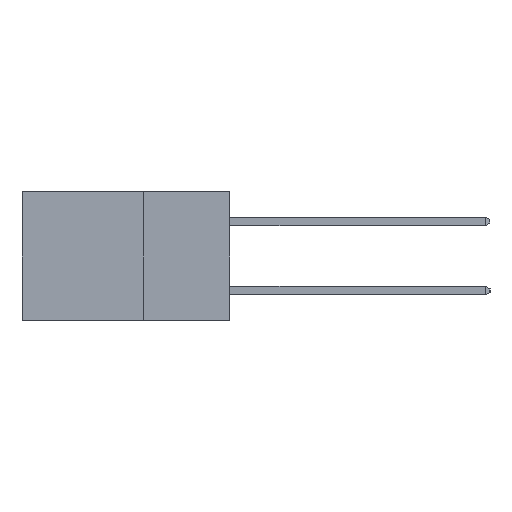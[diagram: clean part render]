
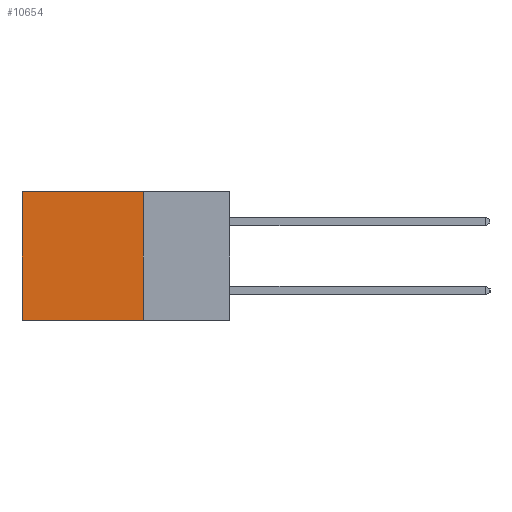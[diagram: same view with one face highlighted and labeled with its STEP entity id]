
A CAD part, left-side view. The second image highlights one B-rep face of the part: STEP entity #10654.
In plain terms, the highlighted planar face has unit normal (-1, 0, 0).
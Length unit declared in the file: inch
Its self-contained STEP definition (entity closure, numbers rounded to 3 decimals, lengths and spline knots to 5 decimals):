
#202 = CARTESIAN_POINT ( 'NONE',  ( 0.2615, 0.25, -0.37 ) ) ;
#442 = DIRECTION ( 'NONE',  ( 0., 0., -1. ) ) ;
#1009 = VERTEX_POINT ( 'NONE', #6782 ) ;
#1456 = DIRECTION ( 'NONE',  ( 1., 0., 0. ) ) ;
#1971 = VECTOR ( 'NONE', #8058, 39.37008 ) ;
#2133 = VERTEX_POINT ( 'NONE', #7729 ) ;
#2610 = CARTESIAN_POINT ( 'NONE',  ( 0.2615, 0.25, -0.37 ) ) ;
#2771 = VECTOR ( 'NONE', #12347, 39.37008 ) ;
#2778 = ORIENTED_EDGE ( 'NONE', *, *, #12112, .F. ) ;
#3104 = VECTOR ( 'NONE', #442, 39.37008 ) ;
#4821 = EDGE_CURVE ( 'NONE', #2133, #5373, #10123, .T. ) ;
#4939 = LINE ( 'NONE', #8272, #1971 ) ;
#5373 = VERTEX_POINT ( 'NONE', #10632 ) ;
#5421 = ORIENTED_EDGE ( 'NONE', *, *, #9676, .T. ) ;
#6753 = CARTESIAN_POINT ( 'NONE',  ( 0.2615, 0.25, -0.37 ) ) ;
#6767 = CARTESIAN_POINT ( 'NONE',  ( 0.2615, 0.25, -0.37 ) ) ;
#6782 = CARTESIAN_POINT ( 'NONE',  ( 0.2615, 0.6, -0.37 ) ) ;
#7162 = VECTOR ( 'NONE', #14064, 39.37008 ) ;
#7729 = CARTESIAN_POINT ( 'NONE',  ( 0.2615, 0.25, 0. ) ) ;
#8058 = DIRECTION ( 'NONE',  ( 0., 0., -1. ) ) ;
#8272 = CARTESIAN_POINT ( 'NONE',  ( 0.2615, 0.6, -0.37 ) ) ;
#8655 = LINE ( 'NONE', #202, #2771 ) ;
#8991 = LINE ( 'NONE', #2610, #3104 ) ;
#9182 = DIRECTION ( 'NONE',  ( 0., 0., -1. ) ) ;
#9676 = EDGE_CURVE ( 'NONE', #5373, #1009, #4939, .T. ) ;
#10123 = LINE ( 'NONE', #14164, #7162 ) ;
#10632 = CARTESIAN_POINT ( 'NONE',  ( 0.2615, 0.6, 0. ) ) ;
#10654 = ADVANCED_FACE ( 'NONE', ( #13957 ), #13351, .F. ) ;
#11232 = EDGE_CURVE ( 'NONE', #13299, #1009, #8655, .T. ) ;
#11600 = ORIENTED_EDGE ( 'NONE', *, *, #4821, .T. ) ;
#12112 = EDGE_CURVE ( 'NONE', #2133, #13299, #8991, .T. ) ;
#12347 = DIRECTION ( 'NONE',  ( 0., 1., 0. ) ) ;
#13287 = AXIS2_PLACEMENT_3D ( 'NONE', #6767, #1456, #9182 ) ;
#13299 = VERTEX_POINT ( 'NONE', #6753 ) ;
#13351 = PLANE ( 'NONE',  #13287 ) ;
#13380 = EDGE_LOOP ( 'NONE', ( #5421, #14096, #2778, #11600 ) ) ;
#13957 = FACE_OUTER_BOUND ( 'NONE', #13380, .T. ) ;
#14064 = DIRECTION ( 'NONE',  ( 0., 1., 0. ) ) ;
#14096 = ORIENTED_EDGE ( 'NONE', *, *, #11232, .F. ) ;
#14164 = CARTESIAN_POINT ( 'NONE',  ( 0.2615, 0.25, 0. ) ) ;
